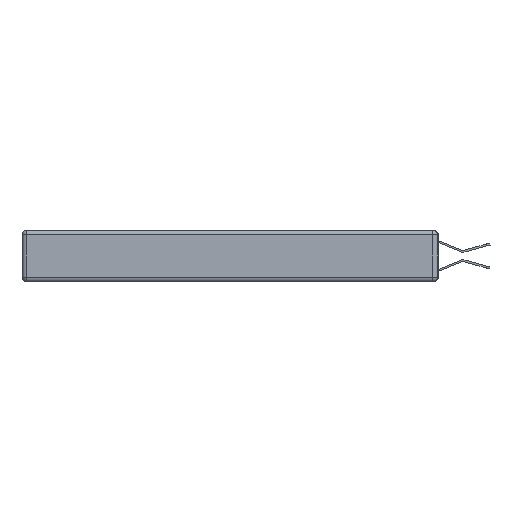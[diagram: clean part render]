
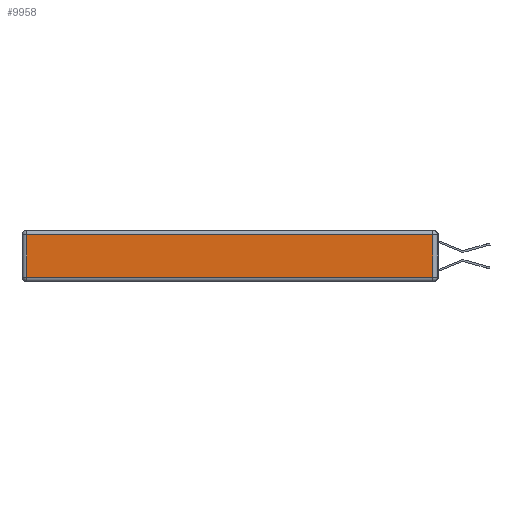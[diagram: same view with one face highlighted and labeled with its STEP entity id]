
A CAD part, left-side view. The second image highlights one B-rep face of the part: STEP entity #9958.
In plain terms, the highlighted planar face has unit normal (-1, 0, 0).
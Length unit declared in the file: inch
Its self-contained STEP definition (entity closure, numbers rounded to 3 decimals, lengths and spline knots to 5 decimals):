
#74 = EDGE_LOOP ( 'NONE', ( #18141, #11088, #7489, #12923 ) ) ;
#1196 = EDGE_CURVE ( 'NONE', #15368, #17050, #18807, .T. ) ;
#1338 = DIRECTION ( 'NONE',  ( -1., 0., 0. ) ) ;
#1406 = VECTOR ( 'NONE', #5503, 39.37008 ) ;
#1656 = EDGE_CURVE ( 'NONE', #19732, #15368, #13533, .T. ) ;
#3350 = CARTESIAN_POINT ( 'NONE',  ( 0., 0.03, -0.03 ) ) ;
#4805 = DIRECTION ( 'NONE',  ( 0., 1., 0. ) ) ;
#5127 = VECTOR ( 'NONE', #21400, 39.37008 ) ;
#5503 = DIRECTION ( 'NONE',  ( 0., -1., 0. ) ) ;
#6407 = VERTEX_POINT ( 'NONE', #11447 ) ;
#6456 = CARTESIAN_POINT ( 'NONE',  ( 0., 0.03, -0.343 ) ) ;
#7192 = VECTOR ( 'NONE', #14903, 39.37008 ) ;
#7489 = ORIENTED_EDGE ( 'NONE', *, *, #1656, .T. ) ;
#8345 = CARTESIAN_POINT ( 'NONE',  ( 0., 2.75, -0.03 ) ) ;
#9627 = LINE ( 'NONE', #6456, #5127 ) ;
#9705 = CARTESIAN_POINT ( 'NONE',  ( 0., 0., -0.343 ) ) ;
#9958 = ADVANCED_FACE ( 'NONE', ( #11799 ), #18097, .T. ) ;
#10414 = LINE ( 'NONE', #15630, #1406 ) ;
#10918 = EDGE_CURVE ( 'NONE', #17050, #6407, #10414, .T. ) ;
#11088 = ORIENTED_EDGE ( 'NONE', *, *, #17357, .T. ) ;
#11181 = CARTESIAN_POINT ( 'NONE',  ( 0., 2.72, -0.03 ) ) ;
#11274 = AXIS2_PLACEMENT_3D ( 'NONE', #9705, #1338, #21466 ) ;
#11447 = CARTESIAN_POINT ( 'NONE',  ( 0., 0.03, -0.313 ) ) ;
#11655 = CARTESIAN_POINT ( 'NONE',  ( 0., 2.72, -0.343 ) ) ;
#11799 = FACE_OUTER_BOUND ( 'NONE', #74, .T. ) ;
#12923 = ORIENTED_EDGE ( 'NONE', *, *, #1196, .T. ) ;
#13533 = LINE ( 'NONE', #8345, #15133 ) ;
#14903 = DIRECTION ( 'NONE',  ( 0., 0., -1. ) ) ;
#15133 = VECTOR ( 'NONE', #4805, 39.37008 ) ;
#15368 = VERTEX_POINT ( 'NONE', #11181 ) ;
#15630 = CARTESIAN_POINT ( 'NONE',  ( 0., 0., -0.313 ) ) ;
#17050 = VERTEX_POINT ( 'NONE', #17584 ) ;
#17357 = EDGE_CURVE ( 'NONE', #6407, #19732, #9627, .T. ) ;
#17584 = CARTESIAN_POINT ( 'NONE',  ( 0., 2.72, -0.313 ) ) ;
#18097 = PLANE ( 'NONE',  #11274 ) ;
#18141 = ORIENTED_EDGE ( 'NONE', *, *, #10918, .T. ) ;
#18807 = LINE ( 'NONE', #11655, #7192 ) ;
#19732 = VERTEX_POINT ( 'NONE', #3350 ) ;
#21400 = DIRECTION ( 'NONE',  ( 0., 0., 1. ) ) ;
#21466 = DIRECTION ( 'NONE',  ( 0., 0., 1. ) ) ;
